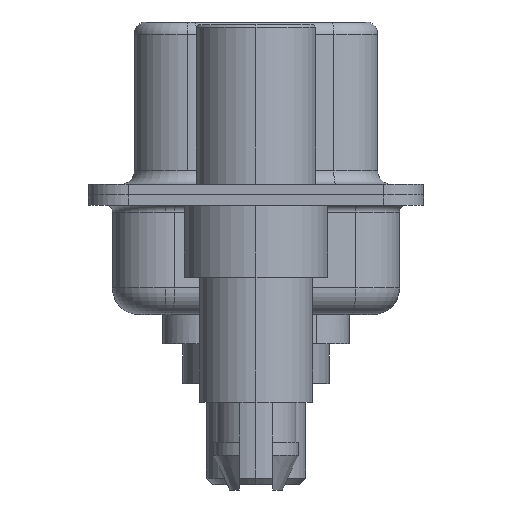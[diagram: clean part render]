
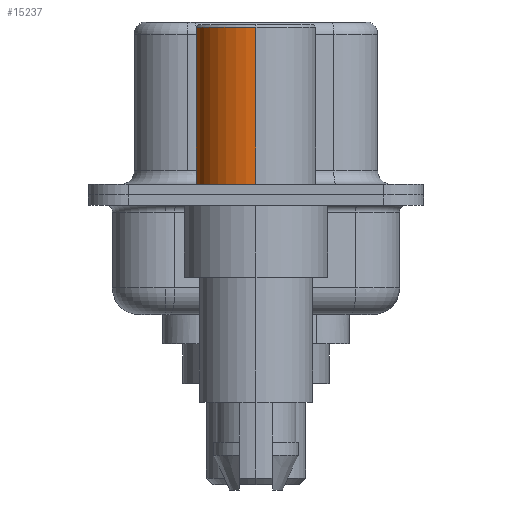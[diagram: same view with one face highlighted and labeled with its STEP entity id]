
A CAD part, left-side view. The second image highlights one B-rep face of the part: STEP entity #15237.
In plain terms, the highlighted cylindrical face has radius 2.25 mm (diameter 4.5 mm), a partial arc.
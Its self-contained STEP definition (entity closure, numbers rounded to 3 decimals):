
#239 = EDGE_CURVE ( 'NONE', #3166, #715, #6133, .T. ) ;
#715 = VERTEX_POINT ( 'NONE', #1438 ) ;
#1438 = CARTESIAN_POINT ( 'NONE',  ( -2.25, 0., 0.4 ) ) ;
#2568 = AXIS2_PLACEMENT_3D ( 'NONE', #5152, #13760, #6410 ) ;
#2639 = CARTESIAN_POINT ( 'NONE',  ( 2.25, 0., 0.4 ) ) ;
#3166 = VERTEX_POINT ( 'NONE', #2639 ) ;
#4158 = EDGE_LOOP ( 'NONE', ( #13841, #10879, #14901, #12007 ) ) ;
#4244 = CARTESIAN_POINT ( 'NONE',  ( 0., 0., 6.3 ) ) ;
#4301 = CARTESIAN_POINT ( 'NONE',  ( -2.25, 0., 6.3 ) ) ;
#4855 = VECTOR ( 'NONE', #7432, 1000. ) ;
#4973 = VERTEX_POINT ( 'NONE', #12894 ) ;
#5152 = CARTESIAN_POINT ( 'NONE',  ( 0., 0., 0.581 ) ) ;
#5403 = DIRECTION ( 'NONE',  ( 0., 0., 1. ) ) ;
#5487 = DIRECTION ( 'NONE',  ( 1., 0., 0. ) ) ;
#5954 = AXIS2_PLACEMENT_3D ( 'NONE', #13618, #5403, #9842 ) ;
#6133 = CIRCLE ( 'NONE', #5954, 2.25 ) ;
#6151 = LINE ( 'NONE', #10070, #12344 ) ;
#6410 = DIRECTION ( 'NONE',  ( 1., 0., 0. ) ) ;
#6799 = CIRCLE ( 'NONE', #8090, 2.25 ) ;
#7255 = VERTEX_POINT ( 'NONE', #4301 ) ;
#7432 = DIRECTION ( 'NONE',  ( 0., 0., 1. ) ) ;
#8090 = AXIS2_PLACEMENT_3D ( 'NONE', #4244, #12870, #5487 ) ;
#9842 = DIRECTION ( 'NONE',  ( 1., 0., 0. ) ) ;
#9948 = CYLINDRICAL_SURFACE ( 'NONE', #2568, 2.25 ) ;
#10070 = CARTESIAN_POINT ( 'NONE',  ( 2.25, 0., 0.581 ) ) ;
#10736 = FACE_OUTER_BOUND ( 'NONE', #4158, .T. ) ;
#10879 = ORIENTED_EDGE ( 'NONE', *, *, #14633, .T. ) ;
#11312 = DIRECTION ( 'NONE',  ( 0., 0., 1. ) ) ;
#11501 = LINE ( 'NONE', #12361, #4855 ) ;
#11687 = EDGE_CURVE ( 'NONE', #4973, #7255, #6799, .T. ) ;
#12007 = ORIENTED_EDGE ( 'NONE', *, *, #13857, .F. ) ;
#12344 = VECTOR ( 'NONE', #11312, 1000. ) ;
#12361 = CARTESIAN_POINT ( 'NONE',  ( -2.25, 0., 0.581 ) ) ;
#12870 = DIRECTION ( 'NONE',  ( 0., 0., 1. ) ) ;
#12894 = CARTESIAN_POINT ( 'NONE',  ( 2.25, 0., 6.3 ) ) ;
#13618 = CARTESIAN_POINT ( 'NONE',  ( 0., 0., 0.4 ) ) ;
#13760 = DIRECTION ( 'NONE',  ( 0., 0., 1. ) ) ;
#13841 = ORIENTED_EDGE ( 'NONE', *, *, #239, .T. ) ;
#13857 = EDGE_CURVE ( 'NONE', #3166, #4973, #6151, .T. ) ;
#14633 = EDGE_CURVE ( 'NONE', #715, #7255, #11501, .T. ) ;
#14901 = ORIENTED_EDGE ( 'NONE', *, *, #11687, .F. ) ;
#15237 = ADVANCED_FACE ( 'NONE', ( #10736 ), #9948, .T. ) ;
